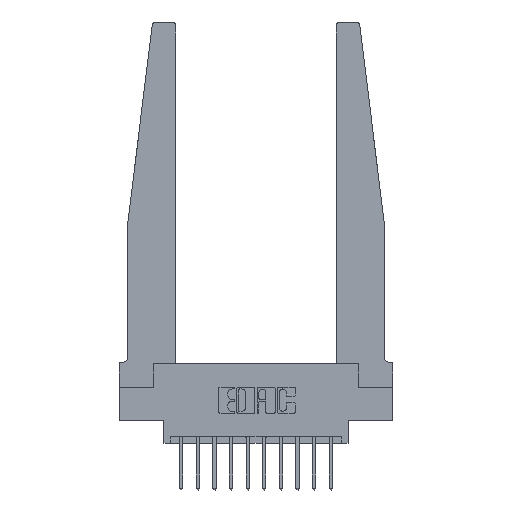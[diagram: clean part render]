
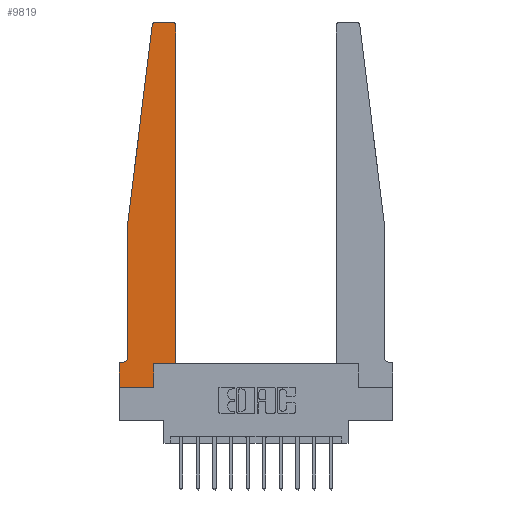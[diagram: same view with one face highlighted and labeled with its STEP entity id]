
A CAD part, top view. The second image highlights one B-rep face of the part: STEP entity #9819.
In plain terms, the highlighted planar face has unit normal (0, 0, 1).
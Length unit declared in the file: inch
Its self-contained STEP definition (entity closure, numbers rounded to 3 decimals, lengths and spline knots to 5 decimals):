
#101 = CARTESIAN_POINT ( 'NONE',  ( 0., 0., 0.37 ) ) ;
#473 = PLANE ( 'NONE',  #2643 ) ;
#605 = CIRCLE ( 'NONE', #14109, 0.03 ) ;
#610 = DIRECTION ( 'NONE',  ( 1., 0., 0. ) ) ;
#796 = EDGE_CURVE ( 'NONE', #13882, #2208, #2233, .T. ) ;
#899 = VERTEX_POINT ( 'NONE', #11554 ) ;
#985 = LINE ( 'NONE', #4336, #10423 ) ;
#1236 = DIRECTION ( 'NONE',  ( 0., 0., 1. ) ) ;
#1350 = VERTEX_POINT ( 'NONE', #2531 ) ;
#1375 = CARTESIAN_POINT ( 'NONE',  ( 0.425, 0.18, 0.37 ) ) ;
#1726 = DIRECTION ( 'NONE',  ( 0., 0., 1. ) ) ;
#1770 = EDGE_CURVE ( 'NONE', #9827, #899, #3741, .T. ) ;
#2208 = VERTEX_POINT ( 'NONE', #6162 ) ;
#2233 = LINE ( 'NONE', #3397, #11619 ) ;
#2471 = CARTESIAN_POINT ( 'NONE',  ( 0.015, 0.2375, 0.37 ) ) ;
#2531 = CARTESIAN_POINT ( 'NONE',  ( 0.425, 2.72, 0.37 ) ) ;
#2643 = AXIS2_PLACEMENT_3D ( 'NONE', #6647, #1726, #10323 ) ;
#2667 = EDGE_LOOP ( 'NONE', ( #6335, #6727, #3008, #5031, #13211, #4149, #6503, #4760, #5159, #6896, #10134, #15716 ) ) ;
#2759 = CIRCLE ( 'NONE', #8036, 0.05 ) ;
#2798 = CARTESIAN_POINT ( 'NONE',  ( 0.395, 2.75, 0.37 ) ) ;
#2840 = DIRECTION ( 'NONE',  ( -1., 0., 0. ) ) ;
#2940 = VECTOR ( 'NONE', #13622, 39.37008 ) ;
#2984 = EDGE_CURVE ( 'NONE', #899, #9771, #5282, .T. ) ;
#3008 = ORIENTED_EDGE ( 'NONE', *, *, #9366, .T. ) ;
#3397 = CARTESIAN_POINT ( 'NONE',  ( 0.2605, 0.18, 0.37 ) ) ;
#3716 = DIRECTION ( 'NONE',  ( -1., 0., 0. ) ) ;
#3741 = LINE ( 'NONE', #7790, #12690 ) ;
#3797 = EDGE_CURVE ( 'NONE', #1350, #13922, #605, .T. ) ;
#3814 = LINE ( 'NONE', #12199, #6749 ) ;
#4014 = CARTESIAN_POINT ( 'NONE',  ( 0.2605, 0., 0.37 ) ) ;
#4064 = CARTESIAN_POINT ( 'NONE',  ( 0., 0., 0.37 ) ) ;
#4149 = ORIENTED_EDGE ( 'NONE', *, *, #1770, .T. ) ;
#4175 = DIRECTION ( 'NONE',  ( 0., -1., 0. ) ) ;
#4336 = CARTESIAN_POINT ( 'NONE',  ( 0.425, 0.18, 0.37 ) ) ;
#4422 = VECTOR ( 'NONE', #4175, 39.37008 ) ;
#4760 = ORIENTED_EDGE ( 'NONE', *, *, #14375, .T. ) ;
#4864 = CARTESIAN_POINT ( 'NONE',  ( 0.065, 1.25, 0.37 ) ) ;
#5031 = ORIENTED_EDGE ( 'NONE', *, *, #5999, .T. ) ;
#5159 = ORIENTED_EDGE ( 'NONE', *, *, #796, .T. ) ;
#5254 = VERTEX_POINT ( 'NONE', #14535 ) ;
#5282 = LINE ( 'NONE', #4064, #12836 ) ;
#5960 = CARTESIAN_POINT ( 'NONE',  ( 0.27653, 2.75, 0.37 ) ) ;
#5999 = EDGE_CURVE ( 'NONE', #12554, #5254, #7711, .T. ) ;
#6162 = CARTESIAN_POINT ( 'NONE',  ( 0.2605, 0.18, 0.37 ) ) ;
#6289 = EDGE_CURVE ( 'NONE', #13922, #6781, #3814, .T. ) ;
#6335 = ORIENTED_EDGE ( 'NONE', *, *, #6289, .T. ) ;
#6407 = EDGE_CURVE ( 'NONE', #10613, #1350, #14446, .T. ) ;
#6503 = ORIENTED_EDGE ( 'NONE', *, *, #2984, .T. ) ;
#6647 = CARTESIAN_POINT ( 'NONE',  ( 0., 0.1875, 0.37 ) ) ;
#6727 = ORIENTED_EDGE ( 'NONE', *, *, #14906, .T. ) ;
#6749 = VECTOR ( 'NONE', #13385, 39.37008 ) ;
#6781 = VERTEX_POINT ( 'NONE', #5960 ) ;
#6896 = ORIENTED_EDGE ( 'NONE', *, *, #10558, .T. ) ;
#7225 = CARTESIAN_POINT ( 'NONE',  ( 0.27653, 2.72, 0.37 ) ) ;
#7655 = CARTESIAN_POINT ( 'NONE',  ( 0.065, 1.25, 0.37 ) ) ;
#7711 = LINE ( 'NONE', #15094, #4422 ) ;
#7790 = CARTESIAN_POINT ( 'NONE',  ( 0.065, 0.1875, 0.37 ) ) ;
#7878 = CARTESIAN_POINT ( 'NONE',  ( 0.015, 0.1875, 0.37 ) ) ;
#8036 = AXIS2_PLACEMENT_3D ( 'NONE', #2471, #11070, #3716 ) ;
#8458 = DIRECTION ( 'NONE',  ( 1., 0., 0. ) ) ;
#8604 = AXIS2_PLACEMENT_3D ( 'NONE', #7225, #15621, #8458 ) ;
#8616 = CARTESIAN_POINT ( 'NONE',  ( 0.395, 2.72, 0.37 ) ) ;
#8671 = EDGE_CURVE ( 'NONE', #5254, #9827, #2759, .T. ) ;
#9115 = VERTEX_POINT ( 'NONE', #14271 ) ;
#9366 = EDGE_CURVE ( 'NONE', #9115, #12554, #12663, .T. ) ;
#9389 = CARTESIAN_POINT ( 'NONE',  ( 0.425, 0.18, 0.37 ) ) ;
#9497 = DIRECTION ( 'NONE',  ( 0., 1., 0. ) ) ;
#9503 = FACE_OUTER_BOUND ( 'NONE', #2667, .T. ) ;
#9771 = VERTEX_POINT ( 'NONE', #13625 ) ;
#9819 = ADVANCED_FACE ( 'NONE', ( #9503 ), #473, .T. ) ;
#9827 = VERTEX_POINT ( 'NONE', #7878 ) ;
#9842 = DIRECTION ( 'NONE',  ( 1., 0., 0. ) ) ;
#9965 = DIRECTION ( 'NONE',  ( 1., 0., 0. ) ) ;
#9997 = LINE ( 'NONE', #101, #12777 ) ;
#10134 = ORIENTED_EDGE ( 'NONE', *, *, #6407, .T. ) ;
#10323 = DIRECTION ( 'NONE',  ( 1., 0., 0. ) ) ;
#10423 = VECTOR ( 'NONE', #610, 39.37008 ) ;
#10558 = EDGE_CURVE ( 'NONE', #2208, #10613, #985, .T. ) ;
#10613 = VERTEX_POINT ( 'NONE', #9389 ) ;
#11070 = DIRECTION ( 'NONE',  ( 0., 0., -1. ) ) ;
#11287 = VECTOR ( 'NONE', #14762, 39.37008 ) ;
#11554 = CARTESIAN_POINT ( 'NONE',  ( 0., 0.1875, 0.37 ) ) ;
#11619 = VECTOR ( 'NONE', #9497, 39.37008 ) ;
#12199 = CARTESIAN_POINT ( 'NONE',  ( 0.25, 2.75, 0.37 ) ) ;
#12554 = VERTEX_POINT ( 'NONE', #4864 ) ;
#12663 = LINE ( 'NONE', #7655, #2940 ) ;
#12690 = VECTOR ( 'NONE', #2840, 39.37008 ) ;
#12761 = CIRCLE ( 'NONE', #8604, 0.03 ) ;
#12777 = VECTOR ( 'NONE', #9965, 39.37008 ) ;
#12836 = VECTOR ( 'NONE', #13772, 39.37008 ) ;
#13211 = ORIENTED_EDGE ( 'NONE', *, *, #8671, .T. ) ;
#13385 = DIRECTION ( 'NONE',  ( -1., 0., 0. ) ) ;
#13622 = DIRECTION ( 'NONE',  ( -0.122, -0.992, 0. ) ) ;
#13625 = CARTESIAN_POINT ( 'NONE',  ( 0., 0., 0.37 ) ) ;
#13772 = DIRECTION ( 'NONE',  ( 0., -1., 0. ) ) ;
#13882 = VERTEX_POINT ( 'NONE', #4014 ) ;
#13922 = VERTEX_POINT ( 'NONE', #2798 ) ;
#14109 = AXIS2_PLACEMENT_3D ( 'NONE', #8616, #1236, #9842 ) ;
#14271 = CARTESIAN_POINT ( 'NONE',  ( 0.24675, 2.72367, 0.37 ) ) ;
#14375 = EDGE_CURVE ( 'NONE', #9771, #13882, #9997, .T. ) ;
#14446 = LINE ( 'NONE', #1375, #11287 ) ;
#14535 = CARTESIAN_POINT ( 'NONE',  ( 0.065, 0.2375, 0.37 ) ) ;
#14762 = DIRECTION ( 'NONE',  ( 0., 1., 0. ) ) ;
#14906 = EDGE_CURVE ( 'NONE', #6781, #9115, #12761, .T. ) ;
#15094 = CARTESIAN_POINT ( 'NONE',  ( 0.065, 1.25, 0.37 ) ) ;
#15621 = DIRECTION ( 'NONE',  ( 0., 0., 1. ) ) ;
#15716 = ORIENTED_EDGE ( 'NONE', *, *, #3797, .T. ) ;
